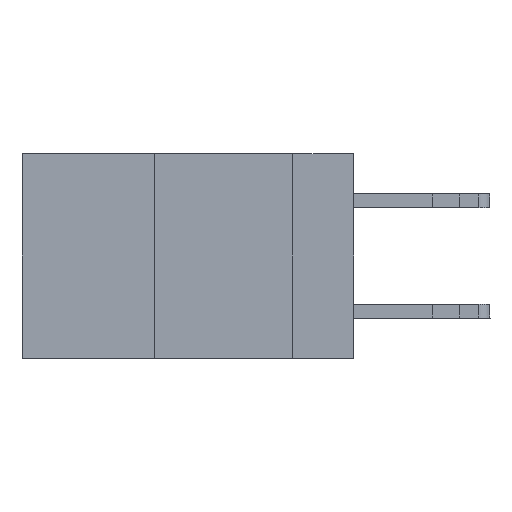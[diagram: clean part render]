
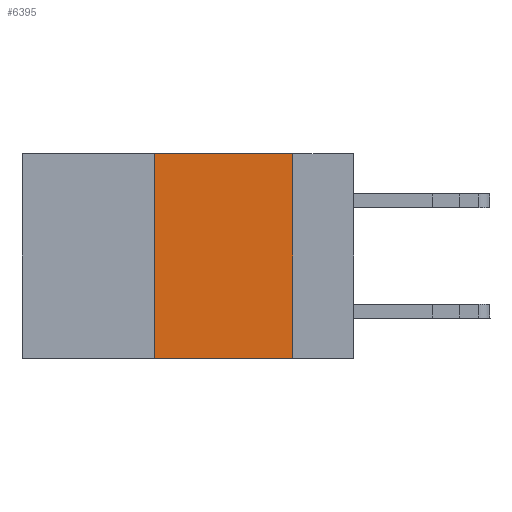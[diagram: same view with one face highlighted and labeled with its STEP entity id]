
A CAD part, left-side view. The second image highlights one B-rep face of the part: STEP entity #6395.
In plain terms, the highlighted planar face has unit normal (-1, 0, 0).
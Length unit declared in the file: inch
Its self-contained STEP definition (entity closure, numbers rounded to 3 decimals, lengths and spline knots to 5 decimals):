
#270 = CARTESIAN_POINT ( 'NONE',  ( 0., 0.11, 0. ) ) ;
#1423 = ORIENTED_EDGE ( 'NONE', *, *, #9145, .F. ) ;
#1924 = EDGE_LOOP ( 'NONE', ( #1423, #16249, #20930, #2540 ) ) ;
#2540 = ORIENTED_EDGE ( 'NONE', *, *, #13967, .T. ) ;
#3711 = LINE ( 'NONE', #270, #22049 ) ;
#3962 = DIRECTION ( 'NONE',  ( 1., 0., 0. ) ) ;
#5552 = DIRECTION ( 'NONE',  ( 0., -1., 0. ) ) ;
#6395 = ADVANCED_FACE ( 'NONE', ( #19975 ), #14718, .F. ) ;
#7507 = VECTOR ( 'NONE', #13664, 39.37008 ) ;
#8917 = AXIS2_PLACEMENT_3D ( 'NONE', #12914, #3962, #16478 ) ;
#9145 = EDGE_CURVE ( 'NONE', #15957, #18286, #3711, .T. ) ;
#10064 = VECTOR ( 'NONE', #16504, 39.37008 ) ;
#10347 = EDGE_CURVE ( 'NONE', #13327, #10836, #19539, .T. ) ;
#10836 = VERTEX_POINT ( 'NONE', #17366 ) ;
#11831 = CARTESIAN_POINT ( 'NONE',  ( 0., 0.6, -0.37 ) ) ;
#12380 = CARTESIAN_POINT ( 'NONE',  ( 0., 0.11, 0. ) ) ;
#12914 = CARTESIAN_POINT ( 'NONE',  ( 0., 0.6, 0. ) ) ;
#13327 = VERTEX_POINT ( 'NONE', #17177 ) ;
#13664 = DIRECTION ( 'NONE',  ( 0., -1., 0. ) ) ;
#13967 = EDGE_CURVE ( 'NONE', #13327, #18286, #16978, .T. ) ;
#14489 = CARTESIAN_POINT ( 'NONE',  ( 0., 0.6, 0. ) ) ;
#14718 = PLANE ( 'NONE',  #8917 ) ;
#15790 = LINE ( 'NONE', #14489, #19911 ) ;
#15957 = VERTEX_POINT ( 'NONE', #12380 ) ;
#16249 = ORIENTED_EDGE ( 'NONE', *, *, #19719, .F. ) ;
#16478 = DIRECTION ( 'NONE',  ( 0., 0., -1. ) ) ;
#16504 = DIRECTION ( 'NONE',  ( 0., 0., 1. ) ) ;
#16978 = LINE ( 'NONE', #11831, #7507 ) ;
#17177 = CARTESIAN_POINT ( 'NONE',  ( 0., 0.36, -0.37 ) ) ;
#17366 = CARTESIAN_POINT ( 'NONE',  ( 0., 0.36, 0. ) ) ;
#18286 = VERTEX_POINT ( 'NONE', #21325 ) ;
#19539 = LINE ( 'NONE', #21365, #10064 ) ;
#19719 = EDGE_CURVE ( 'NONE', #10836, #15957, #15790, .T. ) ;
#19911 = VECTOR ( 'NONE', #5552, 39.37008 ) ;
#19975 = FACE_OUTER_BOUND ( 'NONE', #1924, .T. ) ;
#20930 = ORIENTED_EDGE ( 'NONE', *, *, #10347, .F. ) ;
#21325 = CARTESIAN_POINT ( 'NONE',  ( 0., 0.11, -0.37 ) ) ;
#21365 = CARTESIAN_POINT ( 'NONE',  ( 0., 0.36, 0. ) ) ;
#21713 = DIRECTION ( 'NONE',  ( 0., 0., -1. ) ) ;
#22049 = VECTOR ( 'NONE', #21713, 39.37008 ) ;
